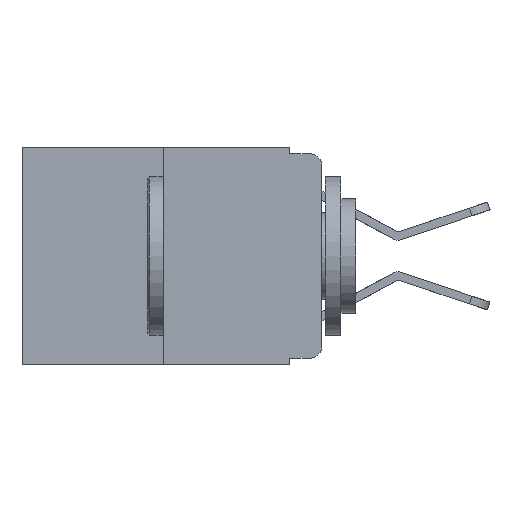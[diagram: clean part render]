
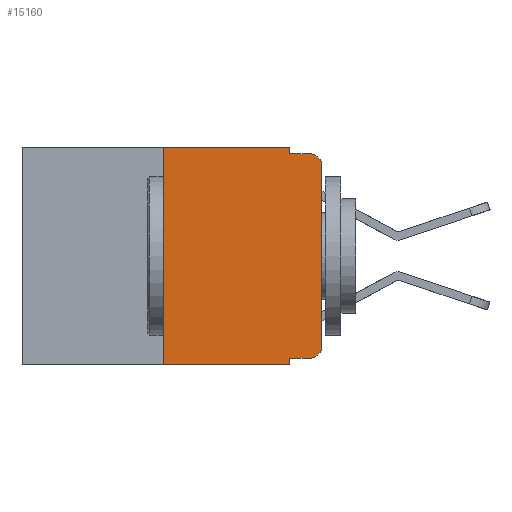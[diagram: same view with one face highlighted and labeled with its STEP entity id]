
A CAD part, left-side view. The second image highlights one B-rep face of the part: STEP entity #15160.
In plain terms, the highlighted planar face has unit normal (-1, 0, 0).
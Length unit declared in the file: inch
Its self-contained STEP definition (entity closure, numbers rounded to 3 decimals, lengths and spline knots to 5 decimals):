
#420 = CARTESIAN_POINT ( 'NONE',  ( 0., 0.051, -0.333 ) ) ;
#573 = CARTESIAN_POINT ( 'NONE',  ( 0., 0.051, -0.01 ) ) ;
#720 = VECTOR ( 'NONE', #12101, 39.37008 ) ;
#770 = VERTEX_POINT ( 'NONE', #3040 ) ;
#1284 = AXIS2_PLACEMENT_3D ( 'NONE', #18085, #1647, #12185 ) ;
#1311 = AXIS2_PLACEMENT_3D ( 'NONE', #11008, #2005, #12532 ) ;
#1647 = DIRECTION ( 'NONE',  ( 1., 0., 0. ) ) ;
#1878 = LINE ( 'NONE', #573, #12937 ) ;
#1901 = EDGE_CURVE ( 'NONE', #2939, #19359, #7589, .T. ) ;
#2005 = DIRECTION ( 'NONE',  ( -1., 0., 0. ) ) ;
#2547 = EDGE_CURVE ( 'NONE', #15341, #7008, #12268, .T. ) ;
#2588 = DIRECTION ( 'NONE',  ( 0., -1., 0. ) ) ;
#2652 = LINE ( 'NONE', #16559, #18102 ) ;
#2749 = CARTESIAN_POINT ( 'NONE',  ( 0., 0.051, 0. ) ) ;
#2772 = LINE ( 'NONE', #5229, #18208 ) ;
#2778 = VERTEX_POINT ( 'NONE', #9331 ) ;
#2939 = VERTEX_POINT ( 'NONE', #420 ) ;
#3040 = CARTESIAN_POINT ( 'NONE',  ( 0., 0.02, -0.333 ) ) ;
#3246 = VERTEX_POINT ( 'NONE', #13605 ) ;
#3516 = EDGE_CURVE ( 'NONE', #770, #19306, #19195, .T. ) ;
#3609 = EDGE_CURVE ( 'NONE', #17706, #3246, #1878, .T. ) ;
#3714 = CARTESIAN_POINT ( 'NONE',  ( 0., 0.051, 0. ) ) ;
#3803 = LINE ( 'NONE', #2749, #11314 ) ;
#4450 = DIRECTION ( 'NONE',  ( 0., -1., 0. ) ) ;
#5229 = CARTESIAN_POINT ( 'NONE',  ( 0., 0.473, 0. ) ) ;
#5302 = EDGE_CURVE ( 'NONE', #7008, #17599, #2772, .T. ) ;
#7008 = VERTEX_POINT ( 'NONE', #15478 ) ;
#7074 = ORIENTED_EDGE ( 'NONE', *, *, #8663, .T. ) ;
#7273 = DIRECTION ( 'NONE',  ( 0., 0., -1. ) ) ;
#7330 = ORIENTED_EDGE ( 'NONE', *, *, #13055, .T. ) ;
#7589 = LINE ( 'NONE', #15950, #19010 ) ;
#7691 = FACE_OUTER_BOUND ( 'NONE', #14033, .T. ) ;
#7953 = DIRECTION ( 'NONE',  ( 0., 0., -1. ) ) ;
#8104 = AXIS2_PLACEMENT_3D ( 'NONE', #14262, #17791, #7953 ) ;
#8663 = EDGE_CURVE ( 'NONE', #19306, #2778, #2652, .T. ) ;
#8945 = CARTESIAN_POINT ( 'NONE',  ( 0., 0.25, 0. ) ) ;
#9331 = CARTESIAN_POINT ( 'NONE',  ( 0., 0., -0.03 ) ) ;
#9470 = ORIENTED_EDGE ( 'NONE', *, *, #11227, .F. ) ;
#9737 = EDGE_CURVE ( 'NONE', #2939, #770, #18152, .T. ) ;
#11008 = CARTESIAN_POINT ( 'NONE',  ( 0., 0.02, -0.03 ) ) ;
#11103 = CARTESIAN_POINT ( 'NONE',  ( 0., 0.25, -0.343 ) ) ;
#11227 = EDGE_CURVE ( 'NONE', #17599, #17706, #3803, .T. ) ;
#11263 = CARTESIAN_POINT ( 'NONE',  ( 0., 0.051, -0.343 ) ) ;
#11314 = VECTOR ( 'NONE', #7273, 39.37008 ) ;
#11452 = CARTESIAN_POINT ( 'NONE',  ( 0., 0.051, -0.01 ) ) ;
#11760 = DIRECTION ( 'NONE',  ( 0., -1., 0. ) ) ;
#11800 = ORIENTED_EDGE ( 'NONE', *, *, #1901, .F. ) ;
#12101 = DIRECTION ( 'NONE',  ( 0., 0., 1. ) ) ;
#12185 = DIRECTION ( 'NONE',  ( 0., 0., -1. ) ) ;
#12268 = LINE ( 'NONE', #8945, #720 ) ;
#12532 = DIRECTION ( 'NONE',  ( 0., 0., -1. ) ) ;
#12678 = LINE ( 'NONE', #13466, #17095 ) ;
#12742 = ORIENTED_EDGE ( 'NONE', *, *, #9737, .T. ) ;
#12937 = VECTOR ( 'NONE', #2588, 39.37008 ) ;
#13055 = EDGE_CURVE ( 'NONE', #15341, #19359, #12678, .T. ) ;
#13466 = CARTESIAN_POINT ( 'NONE',  ( 0., 0.473, -0.343 ) ) ;
#13605 = CARTESIAN_POINT ( 'NONE',  ( 0., 0.02, -0.01 ) ) ;
#13643 = DIRECTION ( 'NONE',  ( 0., 0., 1. ) ) ;
#13917 = ORIENTED_EDGE ( 'NONE', *, *, #2547, .F. ) ;
#14033 = EDGE_LOOP ( 'NONE', ( #7074, #15530, #16460, #9470, #17369, #13917, #7330, #11800, #12742, #16696 ) ) ;
#14233 = VECTOR ( 'NONE', #11760, 39.37008 ) ;
#14262 = CARTESIAN_POINT ( 'NONE',  ( 0., 0.02, -0.313 ) ) ;
#15160 = ADVANCED_FACE ( 'NONE', ( #7691 ), #16604, .F. ) ;
#15341 = VERTEX_POINT ( 'NONE', #11103 ) ;
#15478 = CARTESIAN_POINT ( 'NONE',  ( 0., 0.25, 0. ) ) ;
#15530 = ORIENTED_EDGE ( 'NONE', *, *, #17484, .T. ) ;
#15950 = CARTESIAN_POINT ( 'NONE',  ( 0., 0.051, 0. ) ) ;
#16460 = ORIENTED_EDGE ( 'NONE', *, *, #3609, .F. ) ;
#16559 = CARTESIAN_POINT ( 'NONE',  ( 0., 0., 0. ) ) ;
#16604 = PLANE ( 'NONE',  #1284 ) ;
#16696 = ORIENTED_EDGE ( 'NONE', *, *, #3516, .T. ) ;
#17095 = VECTOR ( 'NONE', #4450, 39.37008 ) ;
#17369 = ORIENTED_EDGE ( 'NONE', *, *, #5302, .F. ) ;
#17398 = CIRCLE ( 'NONE', #1311, 0.02 ) ;
#17484 = EDGE_CURVE ( 'NONE', #2778, #3246, #17398, .T. ) ;
#17599 = VERTEX_POINT ( 'NONE', #3714 ) ;
#17682 = CARTESIAN_POINT ( 'NONE',  ( 0., 0.051, -0.333 ) ) ;
#17706 = VERTEX_POINT ( 'NONE', #11452 ) ;
#17791 = DIRECTION ( 'NONE',  ( -1., 0., 0. ) ) ;
#17874 = DIRECTION ( 'NONE',  ( 0., 0., -1. ) ) ;
#18085 = CARTESIAN_POINT ( 'NONE',  ( 0., 0.473, 0. ) ) ;
#18102 = VECTOR ( 'NONE', #13643, 39.37008 ) ;
#18152 = LINE ( 'NONE', #17682, #14233 ) ;
#18208 = VECTOR ( 'NONE', #18676, 39.37008 ) ;
#18555 = CARTESIAN_POINT ( 'NONE',  ( 0., 0., -0.313 ) ) ;
#18676 = DIRECTION ( 'NONE',  ( 0., -1., 0. ) ) ;
#19010 = VECTOR ( 'NONE', #17874, 39.37008 ) ;
#19195 = CIRCLE ( 'NONE', #8104, 0.02 ) ;
#19306 = VERTEX_POINT ( 'NONE', #18555 ) ;
#19359 = VERTEX_POINT ( 'NONE', #11263 ) ;
